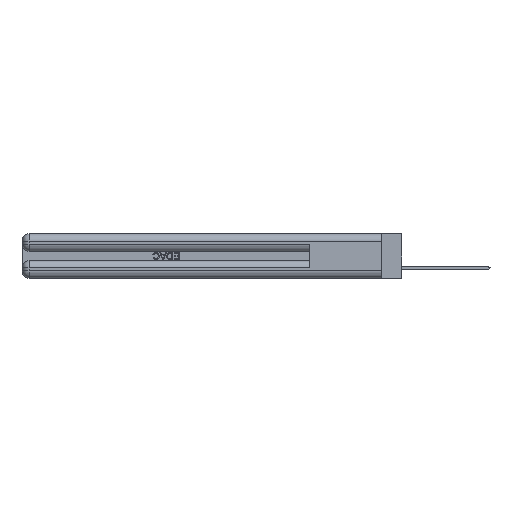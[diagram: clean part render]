
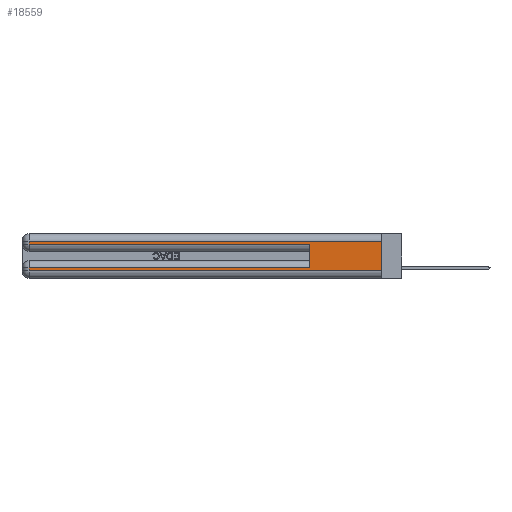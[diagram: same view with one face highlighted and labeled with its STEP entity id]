
A CAD part, left-side view. The second image highlights one B-rep face of the part: STEP entity #18559.
In plain terms, the highlighted planar face has unit normal (-1, 0, 0).
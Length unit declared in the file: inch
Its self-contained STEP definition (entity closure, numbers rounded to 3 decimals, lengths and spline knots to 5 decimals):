
#2635 = EDGE_CURVE ( 'NONE', #30287, #32255, #14117, .T. ) ;
#2770 = CARTESIAN_POINT ( 'NONE',  ( 0., 0., 0.085 ) ) ;
#3124 = VERTEX_POINT ( 'NONE', #25960 ) ;
#3739 = FACE_OUTER_BOUND ( 'NONE', #49067, .T. ) ;
#3743 = ORIENTED_EDGE ( 'NONE', *, *, #2635, .T. ) ;
#4974 = ORIENTED_EDGE ( 'NONE', *, *, #6291, .F. ) ;
#5491 = DIRECTION ( 'NONE',  ( 0., -1., 0. ) ) ;
#5762 = CARTESIAN_POINT ( 'NONE',  ( 0., 0., 0.06 ) ) ;
#6291 = EDGE_CURVE ( 'NONE', #23821, #45005, #40862, .T. ) ;
#6668 = VECTOR ( 'NONE', #5491, 39.37008 ) ;
#9053 = LINE ( 'NONE', #19801, #38798 ) ;
#10572 = VECTOR ( 'NONE', #30219, 39.37008 ) ;
#10924 = CARTESIAN_POINT ( 'NONE',  ( 0., 2.94, 0.06 ) ) ;
#11977 = ORIENTED_EDGE ( 'NONE', *, *, #17996, .F. ) ;
#13200 = CARTESIAN_POINT ( 'NONE',  ( 0., 0., 0.285 ) ) ;
#14075 = CARTESIAN_POINT ( 'NONE',  ( 0., 0.6, 0.085 ) ) ;
#14117 = LINE ( 'NONE', #5762, #34330 ) ;
#15340 = VECTOR ( 'NONE', #47404, 39.37008 ) ;
#15574 = CARTESIAN_POINT ( 'NONE',  ( 0., 0., 0.37 ) ) ;
#17230 = LINE ( 'NONE', #2770, #19812 ) ;
#17234 = ORIENTED_EDGE ( 'NONE', *, *, #51684, .T. ) ;
#17996 = EDGE_CURVE ( 'NONE', #47339, #32255, #44047, .T. ) ;
#18027 = DIRECTION ( 'NONE',  ( 0., 1., 0. ) ) ;
#18559 = ADVANCED_FACE ( 'NONE', ( #3739 ), #43956, .F. ) ;
#19472 = DIRECTION ( 'NONE',  ( 0., 0., -1. ) ) ;
#19529 = EDGE_CURVE ( 'NONE', #23821, #3124, #17230, .T. ) ;
#19801 = CARTESIAN_POINT ( 'NONE',  ( 0., 2.94, 0.37 ) ) ;
#19812 = VECTOR ( 'NONE', #18027, 39.37008 ) ;
#22542 = DIRECTION ( 'NONE',  ( 0., -1., 0. ) ) ;
#23639 = EDGE_CURVE ( 'NONE', #34941, #46352, #47946, .T. ) ;
#23821 = VERTEX_POINT ( 'NONE', #14075 ) ;
#24135 = CARTESIAN_POINT ( 'NONE',  ( 0., 0., 0.37 ) ) ;
#25960 = CARTESIAN_POINT ( 'NONE',  ( 0., 2.94, 0.085 ) ) ;
#26454 = AXIS2_PLACEMENT_3D ( 'NONE', #15574, #47358, #39587 ) ;
#26964 = CARTESIAN_POINT ( 'NONE',  ( 0., 0.6, 0.285 ) ) ;
#28540 = LINE ( 'NONE', #31506, #15340 ) ;
#30094 = VECTOR ( 'NONE', #33921, 39.37008 ) ;
#30219 = DIRECTION ( 'NONE',  ( 0., 0., -1. ) ) ;
#30287 = VERTEX_POINT ( 'NONE', #10924 ) ;
#30800 = CARTESIAN_POINT ( 'NONE',  ( 0., 2.94, 0.37 ) ) ;
#31448 = ORIENTED_EDGE ( 'NONE', *, *, #44065, .T. ) ;
#31506 = CARTESIAN_POINT ( 'NONE',  ( 0., 0., 0.31 ) ) ;
#32255 = VERTEX_POINT ( 'NONE', #36931 ) ;
#33921 = DIRECTION ( 'NONE',  ( 0., 0., 1. ) ) ;
#34330 = VECTOR ( 'NONE', #22542, 39.37008 ) ;
#34941 = VERTEX_POINT ( 'NONE', #46927 ) ;
#36931 = CARTESIAN_POINT ( 'NONE',  ( 0., 0., 0.06 ) ) ;
#37046 = EDGE_CURVE ( 'NONE', #47339, #34941, #28540, .T. ) ;
#37620 = ORIENTED_EDGE ( 'NONE', *, *, #19529, .T. ) ;
#38798 = VECTOR ( 'NONE', #19472, 39.37008 ) ;
#39587 = DIRECTION ( 'NONE',  ( 0., 0., -1. ) ) ;
#40862 = LINE ( 'NONE', #49764, #30094 ) ;
#43956 = PLANE ( 'NONE',  #26454 ) ;
#44047 = LINE ( 'NONE', #24135, #50331 ) ;
#44065 = EDGE_CURVE ( 'NONE', #46352, #45005, #52118, .T. ) ;
#44578 = ORIENTED_EDGE ( 'NONE', *, *, #23639, .T. ) ;
#45005 = VERTEX_POINT ( 'NONE', #26964 ) ;
#45862 = DIRECTION ( 'NONE',  ( 0., 0., -1. ) ) ;
#46101 = CARTESIAN_POINT ( 'NONE',  ( 0., 2.94, 0.285 ) ) ;
#46352 = VERTEX_POINT ( 'NONE', #46101 ) ;
#46927 = CARTESIAN_POINT ( 'NONE',  ( 0., 2.94, 0.31 ) ) ;
#47339 = VERTEX_POINT ( 'NONE', #48395 ) ;
#47358 = DIRECTION ( 'NONE',  ( 1., 0., 0. ) ) ;
#47404 = DIRECTION ( 'NONE',  ( 0., 1., 0. ) ) ;
#47946 = LINE ( 'NONE', #30800, #10572 ) ;
#48395 = CARTESIAN_POINT ( 'NONE',  ( 0., 0., 0.31 ) ) ;
#49067 = EDGE_LOOP ( 'NONE', ( #11977, #51026, #44578, #31448, #4974, #37620, #17234, #3743 ) ) ;
#49764 = CARTESIAN_POINT ( 'NONE',  ( 0., 0.6, 0.145 ) ) ;
#50331 = VECTOR ( 'NONE', #45862, 39.37008 ) ;
#51026 = ORIENTED_EDGE ( 'NONE', *, *, #37046, .T. ) ;
#51684 = EDGE_CURVE ( 'NONE', #3124, #30287, #9053, .T. ) ;
#52118 = LINE ( 'NONE', #13200, #6668 ) ;
